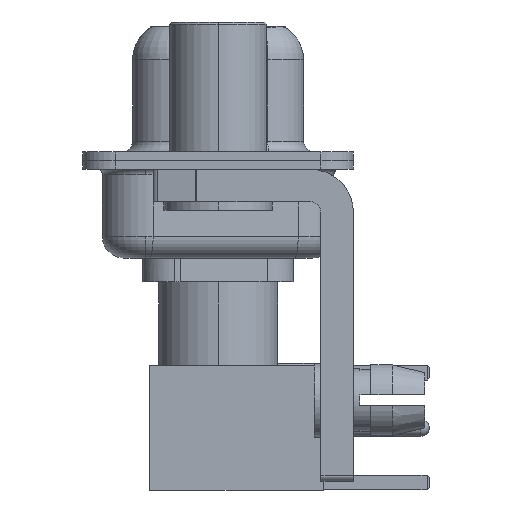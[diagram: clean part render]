
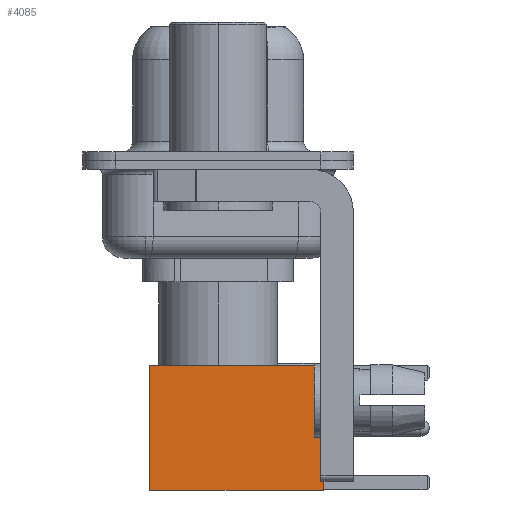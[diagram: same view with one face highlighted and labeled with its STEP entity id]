
A CAD part, left-side view. The second image highlights one B-rep face of the part: STEP entity #4085.
In plain terms, the highlighted face is planar.
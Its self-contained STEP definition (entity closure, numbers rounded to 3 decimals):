
#1201 = DIRECTION ( 'NONE',  ( 0., 0., -1. ) ) ;
#3241 = LINE ( 'NONE', #15841, #20548 ) ;
#3870 = VECTOR ( 'NONE', #9959, 1000. ) ;
#4085 = ADVANCED_FACE ( 'NONE', ( #11067 ), #31196, .T. ) ;
#4170 = ORIENTED_EDGE ( 'NONE', *, *, #13409, .T. ) ;
#4850 = VERTEX_POINT ( 'NONE', #11673 ) ;
#5857 = DIRECTION ( 'NONE',  ( -1., 0., 0. ) ) ;
#7412 = EDGE_LOOP ( 'NONE', ( #23146, #4170, #15201, #29129 ) ) ;
#7475 = EDGE_CURVE ( 'NONE', #4850, #24035, #3241, .T. ) ;
#9222 = LINE ( 'NONE', #21500, #30074 ) ;
#9959 = DIRECTION ( 'NONE',  ( 0., 0., -1. ) ) ;
#10751 = EDGE_CURVE ( 'NONE', #4850, #11313, #9222, .T. ) ;
#11067 = FACE_OUTER_BOUND ( 'NONE', #7412, .T. ) ;
#11313 = VERTEX_POINT ( 'NONE', #13773 ) ;
#11536 = CARTESIAN_POINT ( 'NONE',  ( 0., 2.875, 0. ) ) ;
#11673 = CARTESIAN_POINT ( 'NONE',  ( 2.875, 2.875, 8. ) ) ;
#12413 = CARTESIAN_POINT ( 'NONE',  ( -2.875, 2.875, 0. ) ) ;
#13409 = EDGE_CURVE ( 'NONE', #11313, #26158, #16281, .T. ) ;
#13773 = CARTESIAN_POINT ( 'NONE',  ( 2.875, 2.875, 0. ) ) ;
#14359 = VECTOR ( 'NONE', #28882, 1000. ) ;
#15201 = ORIENTED_EDGE ( 'NONE', *, *, #26686, .F. ) ;
#15770 = CARTESIAN_POINT ( 'NONE',  ( -2.875, 2.875, 0. ) ) ;
#15805 = CARTESIAN_POINT ( 'NONE',  ( 2.875, 2.875, 0. ) ) ;
#15841 = CARTESIAN_POINT ( 'NONE',  ( 0., 2.875, 8. ) ) ;
#16281 = LINE ( 'NONE', #11536, #14359 ) ;
#17947 = DIRECTION ( 'NONE',  ( 0., 0., 1. ) ) ;
#18274 = AXIS2_PLACEMENT_3D ( 'NONE', #15805, #26133, #17947 ) ;
#20266 = LINE ( 'NONE', #12413, #3870 ) ;
#20548 = VECTOR ( 'NONE', #5857, 1000. ) ;
#21500 = CARTESIAN_POINT ( 'NONE',  ( 2.875, 2.875, 0. ) ) ;
#23146 = ORIENTED_EDGE ( 'NONE', *, *, #10751, .T. ) ;
#24035 = VERTEX_POINT ( 'NONE', #27451 ) ;
#26133 = DIRECTION ( 'NONE',  ( 0., 1., 0. ) ) ;
#26158 = VERTEX_POINT ( 'NONE', #15770 ) ;
#26686 = EDGE_CURVE ( 'NONE', #24035, #26158, #20266, .T. ) ;
#27451 = CARTESIAN_POINT ( 'NONE',  ( -2.875, 2.875, 8. ) ) ;
#28882 = DIRECTION ( 'NONE',  ( -1., 0., 0. ) ) ;
#29129 = ORIENTED_EDGE ( 'NONE', *, *, #7475, .F. ) ;
#30074 = VECTOR ( 'NONE', #1201, 1000. ) ;
#31196 = PLANE ( 'NONE',  #18274 ) ;
